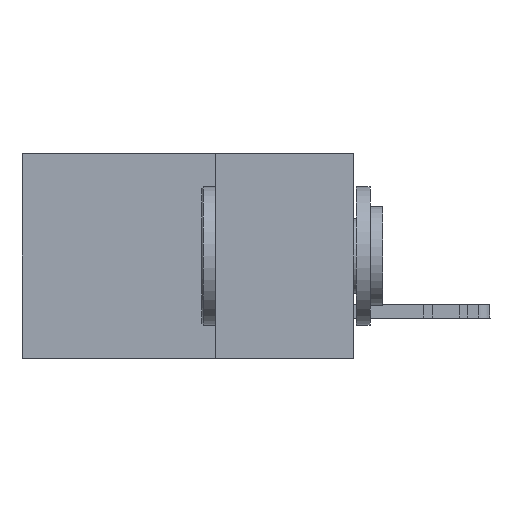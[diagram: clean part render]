
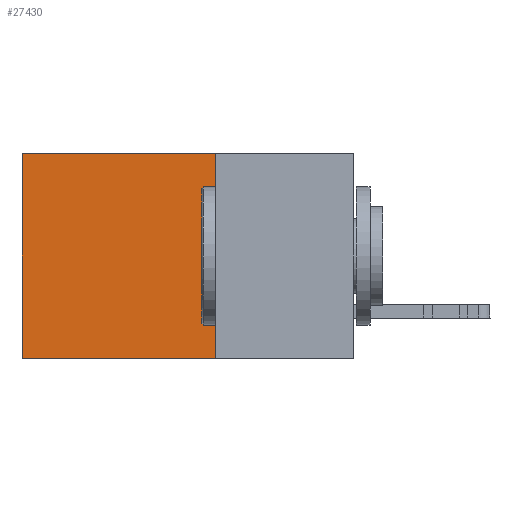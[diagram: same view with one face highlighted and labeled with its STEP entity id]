
A CAD part, left-side view. The second image highlights one B-rep face of the part: STEP entity #27430.
In plain terms, the highlighted planar face has unit normal (-1, 0, 0).
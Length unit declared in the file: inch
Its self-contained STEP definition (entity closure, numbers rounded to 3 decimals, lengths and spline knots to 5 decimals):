
#1551 = ORIENTED_EDGE ( 'NONE', *, *, #31302, .F. ) ;
#3525 = DIRECTION ( 'NONE',  ( 0., 1., 0. ) ) ;
#3699 = VERTEX_POINT ( 'NONE', #27638 ) ;
#6583 = VECTOR ( 'NONE', #3525, 39.37008 ) ;
#7093 = DIRECTION ( 'NONE',  ( 0., 1., 0. ) ) ;
#7992 = CARTESIAN_POINT ( 'NONE',  ( 0.2875, 0.6, -0.37 ) ) ;
#9794 = ORIENTED_EDGE ( 'NONE', *, *, #27155, .T. ) ;
#11520 = CARTESIAN_POINT ( 'NONE',  ( 0.2875, 0.25, 0. ) ) ;
#11912 = EDGE_CURVE ( 'NONE', #3699, #31138, #19196, .T. ) ;
#12301 = VECTOR ( 'NONE', #32866, 39.37008 ) ;
#12318 = CARTESIAN_POINT ( 'NONE',  ( 0.2875, 0.25, 0. ) ) ;
#12721 = VECTOR ( 'NONE', #7093, 39.37008 ) ;
#14786 = CARTESIAN_POINT ( 'NONE',  ( 0.2875, 0.25, 0. ) ) ;
#15961 = DIRECTION ( 'NONE',  ( 0., 0., -1. ) ) ;
#17142 = LINE ( 'NONE', #18035, #35004 ) ;
#18035 = CARTESIAN_POINT ( 'NONE',  ( 0.2875, 0.25, 0. ) ) ;
#19196 = LINE ( 'NONE', #40124, #6583 ) ;
#20201 = AXIS2_PLACEMENT_3D ( 'NONE', #12318, #37962, #15961 ) ;
#20867 = LINE ( 'NONE', #24986, #12301 ) ;
#22460 = LINE ( 'NONE', #14786, #12721 ) ;
#23673 = EDGE_LOOP ( 'NONE', ( #9794, #46822, #1551, #27729 ) ) ;
#24986 = CARTESIAN_POINT ( 'NONE',  ( 0.2875, 0.6, 0. ) ) ;
#25503 = CARTESIAN_POINT ( 'NONE',  ( 0.2875, 0.6, 0. ) ) ;
#26605 = PLANE ( 'NONE',  #20201 ) ;
#27155 = EDGE_CURVE ( 'NONE', #43426, #31138, #20867, .T. ) ;
#27430 = ADVANCED_FACE ( 'NONE', ( #35252 ), #26605, .F. ) ;
#27638 = CARTESIAN_POINT ( 'NONE',  ( 0.2875, 0.25, -0.37 ) ) ;
#27729 = ORIENTED_EDGE ( 'NONE', *, *, #28589, .T. ) ;
#28589 = EDGE_CURVE ( 'NONE', #39731, #43426, #22460, .T. ) ;
#31138 = VERTEX_POINT ( 'NONE', #7992 ) ;
#31302 = EDGE_CURVE ( 'NONE', #39731, #3699, #17142, .T. ) ;
#32866 = DIRECTION ( 'NONE',  ( 0., 0., -1. ) ) ;
#35004 = VECTOR ( 'NONE', #36830, 39.37008 ) ;
#35252 = FACE_OUTER_BOUND ( 'NONE', #23673, .T. ) ;
#36830 = DIRECTION ( 'NONE',  ( 0., 0., -1. ) ) ;
#37962 = DIRECTION ( 'NONE',  ( 1., 0., 0. ) ) ;
#39731 = VERTEX_POINT ( 'NONE', #11520 ) ;
#40124 = CARTESIAN_POINT ( 'NONE',  ( 0.2875, 0.25, -0.37 ) ) ;
#43426 = VERTEX_POINT ( 'NONE', #25503 ) ;
#46822 = ORIENTED_EDGE ( 'NONE', *, *, #11912, .F. ) ;
